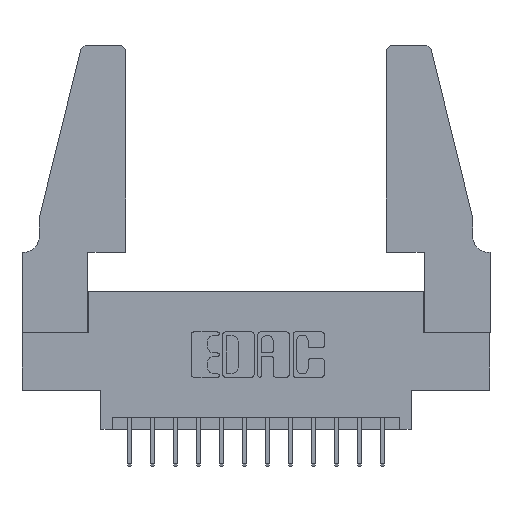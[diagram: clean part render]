
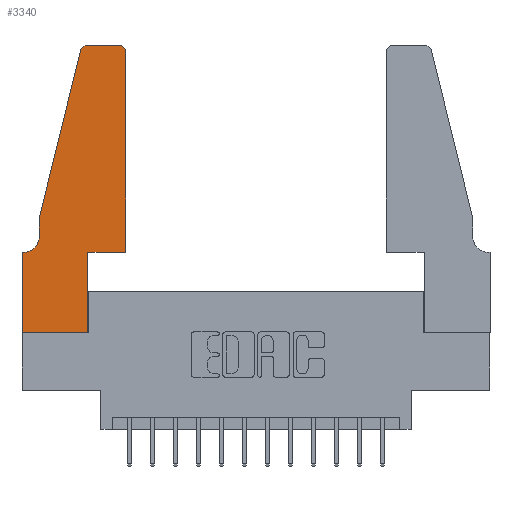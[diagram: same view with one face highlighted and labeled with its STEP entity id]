
A CAD part, top view. The second image highlights one B-rep face of the part: STEP entity #3340.
In plain terms, the highlighted planar face has unit normal (0, 0, 1).
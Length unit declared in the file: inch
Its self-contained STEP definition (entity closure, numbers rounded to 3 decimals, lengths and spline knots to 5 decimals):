
#110 = EDGE_CURVE ( 'NONE', #13391, #13504, #14576, .T. ) ;
#179 = ORIENTED_EDGE ( 'NONE', *, *, #2371, .T. ) ;
#185 = VECTOR ( 'NONE', #9761, 39.37008 ) ;
#372 = VERTEX_POINT ( 'NONE', #1908 ) ;
#685 = DIRECTION ( 'NONE',  ( 1., 0., 0. ) ) ;
#860 = VERTEX_POINT ( 'NONE', #6814 ) ;
#970 = VERTEX_POINT ( 'NONE', #11411 ) ;
#1063 = CARTESIAN_POINT ( 'NONE',  ( 0.0755, 0.5, 0.37 ) ) ;
#1384 = ORIENTED_EDGE ( 'NONE', *, *, #13543, .T. ) ;
#1711 = LINE ( 'NONE', #12176, #8762 ) ;
#1908 = CARTESIAN_POINT ( 'NONE',  ( 0.2865, 0., 0.37 ) ) ;
#2245 = ORIENTED_EDGE ( 'NONE', *, *, #3722, .T. ) ;
#2358 = DIRECTION ( 'NONE',  ( 0., 1., 0. ) ) ;
#2371 = EDGE_CURVE ( 'NONE', #970, #2444, #14260, .T. ) ;
#2444 = VERTEX_POINT ( 'NONE', #9247 ) ;
#2449 = CARTESIAN_POINT ( 'NONE',  ( 0., 0.35, 0.37 ) ) ;
#2804 = LINE ( 'NONE', #15337, #12557 ) ;
#3232 = CARTESIAN_POINT ( 'NONE',  ( 0., 0.35, 0.37 ) ) ;
#3340 = ADVANCED_FACE ( 'NONE', ( #8119 ), #12256, .T. ) ;
#3722 = EDGE_CURVE ( 'NONE', #372, #7266, #15173, .T. ) ;
#3807 = ORIENTED_EDGE ( 'NONE', *, *, #6157, .T. ) ;
#3947 = LINE ( 'NONE', #8613, #10112 ) ;
#4097 = EDGE_LOOP ( 'NONE', ( #10991, #14050, #179, #1384, #9457, #10608, #13858, #11655, #2245, #8908, #5971, #3807 ) ) ;
#4449 = CARTESIAN_POINT ( 'NONE',  ( 0.2865, 0.35, 0.37 ) ) ;
#4492 = CARTESIAN_POINT ( 'NONE',  ( 0.284, 1.25, 0.37 ) ) ;
#4715 = CARTESIAN_POINT ( 'NONE',  ( 0.284, 1.22, 0.37 ) ) ;
#4984 = DIRECTION ( 'NONE',  ( 0., 0., 1. ) ) ;
#5340 = EDGE_CURVE ( 'NONE', #7266, #860, #12506, .T. ) ;
#5521 = AXIS2_PLACEMENT_3D ( 'NONE', #2449, #4984, #13468 ) ;
#5725 = DIRECTION ( 'NONE',  ( 0., 0., -1. ) ) ;
#5896 = AXIS2_PLACEMENT_3D ( 'NONE', #4715, #13217, #5948 ) ;
#5899 = CARTESIAN_POINT ( 'NONE',  ( 0., 0., 0.37 ) ) ;
#5948 = DIRECTION ( 'NONE',  ( 1., 0., 0. ) ) ;
#5971 = ORIENTED_EDGE ( 'NONE', *, *, #14280, .T. ) ;
#6157 = EDGE_CURVE ( 'NONE', #14027, #9737, #9694, .T. ) ;
#6252 = EDGE_CURVE ( 'NONE', #10253, #7383, #14536, .T. ) ;
#6781 = CARTESIAN_POINT ( 'NONE',  ( 0.4205, 1.22, 0.37 ) ) ;
#6814 = CARTESIAN_POINT ( 'NONE',  ( 0.4505, 0.35, 0.37 ) ) ;
#6898 = CARTESIAN_POINT ( 'NONE',  ( 0.4505, 1.22, 0.37 ) ) ;
#7266 = VERTEX_POINT ( 'NONE', #8954 ) ;
#7383 = VERTEX_POINT ( 'NONE', #15120 ) ;
#7875 = AXIS2_PLACEMENT_3D ( 'NONE', #6781, #15166, #8041 ) ;
#7920 = VECTOR ( 'NONE', #11098, 39.37008 ) ;
#8041 = DIRECTION ( 'NONE',  ( 1., 0., 0. ) ) ;
#8119 = FACE_OUTER_BOUND ( 'NONE', #4097, .T. ) ;
#8215 = DIRECTION ( 'NONE',  ( 0., 1., 0. ) ) ;
#8273 = CARTESIAN_POINT ( 'NONE',  ( 0., 0., 0.37 ) ) ;
#8613 = CARTESIAN_POINT ( 'NONE',  ( 0.0755, 0.35, 0.37 ) ) ;
#8762 = VECTOR ( 'NONE', #2358, 39.37008 ) ;
#8908 = ORIENTED_EDGE ( 'NONE', *, *, #5340, .T. ) ;
#8948 = EDGE_CURVE ( 'NONE', #11104, #970, #12252, .T. ) ;
#8954 = CARTESIAN_POINT ( 'NONE',  ( 0.2865, 0.35, 0.37 ) ) ;
#9082 = DIRECTION ( 'NONE',  ( -1., 0., 0. ) ) ;
#9247 = CARTESIAN_POINT ( 'NONE',  ( 0.0755, 0.5, 0.37 ) ) ;
#9370 = VECTOR ( 'NONE', #11070, 39.37008 ) ;
#9457 = ORIENTED_EDGE ( 'NONE', *, *, #6252, .T. ) ;
#9672 = LINE ( 'NONE', #14998, #13225 ) ;
#9694 = CIRCLE ( 'NONE', #7875, 0.03 ) ;
#9737 = VERTEX_POINT ( 'NONE', #15264 ) ;
#9761 = DIRECTION ( 'NONE',  ( 0., -1., 0. ) ) ;
#9810 = DIRECTION ( 'NONE',  ( 0., -1., 0. ) ) ;
#9871 = CARTESIAN_POINT ( 'NONE',  ( 0.4505, 0.35, 0.37 ) ) ;
#10112 = VECTOR ( 'NONE', #12178, 39.37008 ) ;
#10253 = VERTEX_POINT ( 'NONE', #10260 ) ;
#10260 = CARTESIAN_POINT ( 'NONE',  ( 0.0755, 0.42, 0.37 ) ) ;
#10294 = AXIS2_PLACEMENT_3D ( 'NONE', #12996, #5725, #14170 ) ;
#10608 = ORIENTED_EDGE ( 'NONE', *, *, #12332, .T. ) ;
#10991 = ORIENTED_EDGE ( 'NONE', *, *, #14389, .T. ) ;
#11029 = VECTOR ( 'NONE', #9810, 39.37008 ) ;
#11070 = DIRECTION ( 'NONE',  ( 1., 0., 0. ) ) ;
#11086 = EDGE_CURVE ( 'NONE', #13504, #372, #2804, .T. ) ;
#11098 = DIRECTION ( 'NONE',  ( -0.239, -0.971, 0. ) ) ;
#11104 = VERTEX_POINT ( 'NONE', #4492 ) ;
#11223 = CARTESIAN_POINT ( 'NONE',  ( 0.0755, 0.5, 0.37 ) ) ;
#11411 = CARTESIAN_POINT ( 'NONE',  ( 0.25487, 1.22718, 0.37 ) ) ;
#11632 = VECTOR ( 'NONE', #8215, 39.37008 ) ;
#11655 = ORIENTED_EDGE ( 'NONE', *, *, #11086, .T. ) ;
#12176 = CARTESIAN_POINT ( 'NONE',  ( 0.4505, 0.35, 0.37 ) ) ;
#12178 = DIRECTION ( 'NONE',  ( -1., 0., 0. ) ) ;
#12252 = CIRCLE ( 'NONE', #5896, 0.03 ) ;
#12256 = PLANE ( 'NONE',  #5521 ) ;
#12332 = EDGE_CURVE ( 'NONE', #7383, #13391, #3947, .T. ) ;
#12506 = LINE ( 'NONE', #9871, #9370 ) ;
#12557 = VECTOR ( 'NONE', #685, 39.37008 ) ;
#12996 = CARTESIAN_POINT ( 'NONE',  ( 0.0055, 0.42, 0.37 ) ) ;
#13217 = DIRECTION ( 'NONE',  ( 0., 0., 1. ) ) ;
#13225 = VECTOR ( 'NONE', #9082, 39.37008 ) ;
#13391 = VERTEX_POINT ( 'NONE', #3232 ) ;
#13468 = DIRECTION ( 'NONE',  ( 1., 0., 0. ) ) ;
#13504 = VERTEX_POINT ( 'NONE', #5899 ) ;
#13543 = EDGE_CURVE ( 'NONE', #2444, #10253, #15677, .T. ) ;
#13858 = ORIENTED_EDGE ( 'NONE', *, *, #110, .T. ) ;
#14027 = VERTEX_POINT ( 'NONE', #6898 ) ;
#14050 = ORIENTED_EDGE ( 'NONE', *, *, #8948, .T. ) ;
#14170 = DIRECTION ( 'NONE',  ( -1., 0., 0. ) ) ;
#14260 = LINE ( 'NONE', #11223, #7920 ) ;
#14280 = EDGE_CURVE ( 'NONE', #860, #14027, #1711, .T. ) ;
#14389 = EDGE_CURVE ( 'NONE', #9737, #11104, #9672, .T. ) ;
#14536 = CIRCLE ( 'NONE', #10294, 0.07 ) ;
#14576 = LINE ( 'NONE', #8273, #11029 ) ;
#14998 = CARTESIAN_POINT ( 'NONE',  ( 0.2605, 1.25, 0.37 ) ) ;
#15120 = CARTESIAN_POINT ( 'NONE',  ( 0.0055, 0.35, 0.37 ) ) ;
#15166 = DIRECTION ( 'NONE',  ( 0., 0., 1. ) ) ;
#15173 = LINE ( 'NONE', #4449, #11632 ) ;
#15264 = CARTESIAN_POINT ( 'NONE',  ( 0.4205, 1.25, 0.37 ) ) ;
#15337 = CARTESIAN_POINT ( 'NONE',  ( 0., 0., 0.37 ) ) ;
#15677 = LINE ( 'NONE', #1063, #185 ) ;
